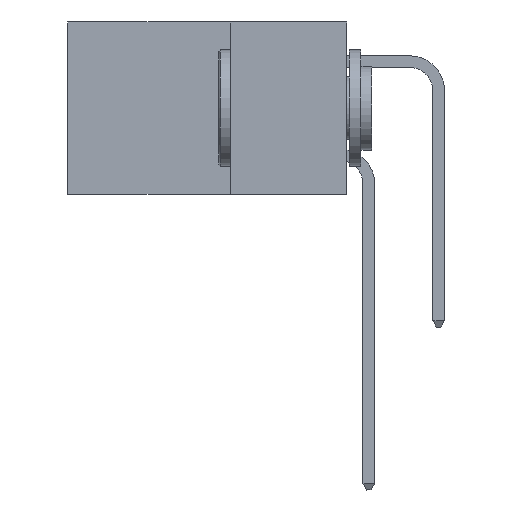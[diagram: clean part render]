
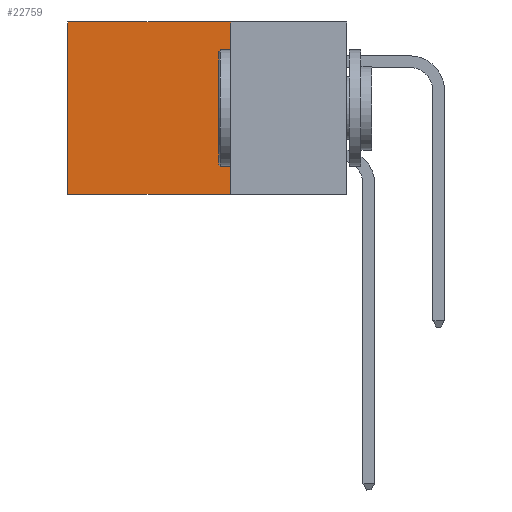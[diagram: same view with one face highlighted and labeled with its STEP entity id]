
A CAD part, left-side view. The second image highlights one B-rep face of the part: STEP entity #22759.
In plain terms, the highlighted planar face has unit normal (-1, 0, 0).
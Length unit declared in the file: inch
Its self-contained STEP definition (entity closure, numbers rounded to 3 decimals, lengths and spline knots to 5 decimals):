
#125 = DIRECTION ( 'NONE',  ( 0., 0., -1. ) ) ;
#248 = CARTESIAN_POINT ( 'NONE',  ( 0.2875, 0.25, -0.37 ) ) ;
#1793 = AXIS2_PLACEMENT_3D ( 'NONE', #10213, #31643, #13324 ) ;
#3342 = VECTOR ( 'NONE', #23516, 39.37008 ) ;
#3900 = CARTESIAN_POINT ( 'NONE',  ( 0.2875, 0.6, -0.37 ) ) ;
#4033 = EDGE_CURVE ( 'NONE', #38771, #7075, #27890, .T. ) ;
#5637 = ORIENTED_EDGE ( 'NONE', *, *, #34390, .T. ) ;
#7013 = DIRECTION ( 'NONE',  ( 0., 0., -1. ) ) ;
#7075 = VERTEX_POINT ( 'NONE', #3900 ) ;
#8489 = ORIENTED_EDGE ( 'NONE', *, *, #4033, .F. ) ;
#10213 = CARTESIAN_POINT ( 'NONE',  ( 0.2875, 0.25, 0. ) ) ;
#10387 = VERTEX_POINT ( 'NONE', #24688 ) ;
#11374 = EDGE_LOOP ( 'NONE', ( #5637, #8489, #20157, #18575 ) ) ;
#11580 = VECTOR ( 'NONE', #19960, 39.37008 ) ;
#12005 = VECTOR ( 'NONE', #7013, 39.37008 ) ;
#12648 = LINE ( 'NONE', #35537, #3342 ) ;
#13324 = DIRECTION ( 'NONE',  ( 0., 0., -1. ) ) ;
#15729 = CARTESIAN_POINT ( 'NONE',  ( 0.2875, 0.25, 0. ) ) ;
#16151 = LINE ( 'NONE', #15729, #31420 ) ;
#18575 = ORIENTED_EDGE ( 'NONE', *, *, #39064, .T. ) ;
#19960 = DIRECTION ( 'NONE',  ( 0., 1., 0. ) ) ;
#20157 = ORIENTED_EDGE ( 'NONE', *, *, #21468, .F. ) ;
#21468 = EDGE_CURVE ( 'NONE', #29717, #38771, #16151, .T. ) ;
#22759 = ADVANCED_FACE ( 'NONE', ( #26091 ), #25547, .F. ) ;
#23516 = DIRECTION ( 'NONE',  ( 0., 1., 0. ) ) ;
#24688 = CARTESIAN_POINT ( 'NONE',  ( 0.2875, 0.6, 0. ) ) ;
#25510 = CARTESIAN_POINT ( 'NONE',  ( 0.2875, 0.6, 0. ) ) ;
#25547 = PLANE ( 'NONE',  #1793 ) ;
#26091 = FACE_OUTER_BOUND ( 'NONE', #11374, .T. ) ;
#27737 = CARTESIAN_POINT ( 'NONE',  ( 0.2875, 0.25, 0. ) ) ;
#27890 = LINE ( 'NONE', #29119, #11580 ) ;
#29119 = CARTESIAN_POINT ( 'NONE',  ( 0.2875, 0.25, -0.37 ) ) ;
#29717 = VERTEX_POINT ( 'NONE', #27737 ) ;
#31420 = VECTOR ( 'NONE', #125, 39.37008 ) ;
#31643 = DIRECTION ( 'NONE',  ( 1., 0., 0. ) ) ;
#34390 = EDGE_CURVE ( 'NONE', #10387, #7075, #35417, .T. ) ;
#35417 = LINE ( 'NONE', #25510, #12005 ) ;
#35537 = CARTESIAN_POINT ( 'NONE',  ( 0.2875, 0.25, 0. ) ) ;
#38771 = VERTEX_POINT ( 'NONE', #248 ) ;
#39064 = EDGE_CURVE ( 'NONE', #29717, #10387, #12648, .T. ) ;
